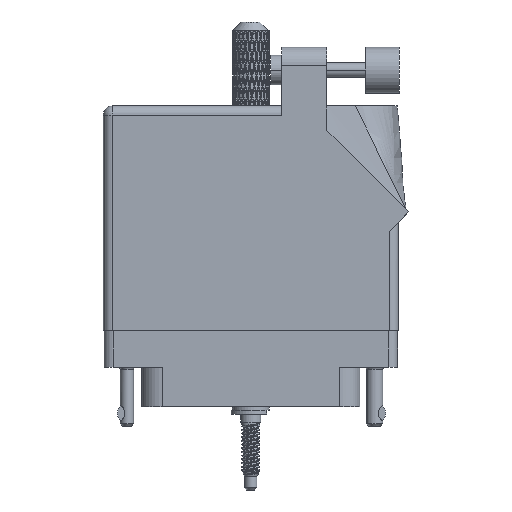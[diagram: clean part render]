
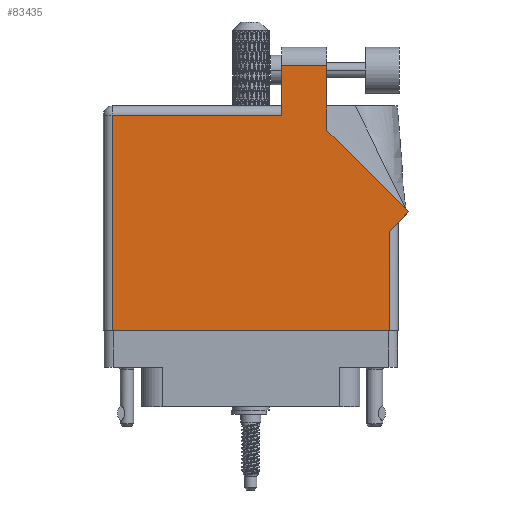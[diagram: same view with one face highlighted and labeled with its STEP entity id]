
A CAD part, front view. The second image highlights one B-rep face of the part: STEP entity #83435.
In plain terms, the highlighted face is planar.
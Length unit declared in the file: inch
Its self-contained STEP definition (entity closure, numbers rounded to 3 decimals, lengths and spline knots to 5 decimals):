
#87 = DIRECTION ( 'NONE',  ( 0., 0., -1. ) ) ;
#1238 = CARTESIAN_POINT ( 'NONE',  ( -0.943, 1.368, 0.455 ) ) ;
#1897 = VERTEX_POINT ( 'NONE', #28675 ) ;
#4050 = VERTEX_POINT ( 'NONE', #73638 ) ;
#4842 = EDGE_CURVE ( 'NONE', #1897, #29199, #67476, .T. ) ;
#5436 = DIRECTION ( 'NONE',  ( 0., 1., 0. ) ) ;
#7036 = ORIENTED_EDGE ( 'NONE', *, *, #47555, .T. ) ;
#7184 = LINE ( 'NONE', #101073, #16944 ) ;
#7627 = LINE ( 'NONE', #17118, #114527 ) ;
#7717 = DIRECTION ( 'NONE',  ( 0.707, 0.707, 0. ) ) ;
#9039 = VECTOR ( 'NONE', #5436, 39.37008 ) ;
#9808 = CARTESIAN_POINT ( 'NONE',  ( -1.005, 1.43, 0.455 ) ) ;
#15026 = VECTOR ( 'NONE', #84404, 39.37008 ) ;
#16944 = VECTOR ( 'NONE', #48210, 39.37008 ) ;
#17118 = CARTESIAN_POINT ( 'NONE',  ( 0.212, 1.43, 0.455 ) ) ;
#23629 = DIRECTION ( 'NONE',  ( 0., 1., 0. ) ) ;
#24159 = VERTEX_POINT ( 'NONE', #89718 ) ;
#24537 = EDGE_LOOP ( 'NONE', ( #7036, #66713, #81963, #40943, #89921, #25358, #95465, #99222, #57016 ) ) ;
#25358 = ORIENTED_EDGE ( 'NONE', *, *, #101197, .T. ) ;
#25859 = EDGE_CURVE ( 'NONE', #4050, #98365, #52923, .T. ) ;
#28675 = CARTESIAN_POINT ( 'NONE',  ( 0.212, 1.368, 0.455 ) ) ;
#29199 = VERTEX_POINT ( 'NONE', #1238 ) ;
#29390 = VERTEX_POINT ( 'NONE', #30710 ) ;
#29556 = EDGE_CURVE ( 'NONE', #29390, #1897, #7627, .T. ) ;
#30710 = CARTESIAN_POINT ( 'NONE',  ( 0.212, 1.705, 0.455 ) ) ;
#32322 = EDGE_CURVE ( 'NONE', #98365, #46793, #7184, .T. ) ;
#33347 = EDGE_CURVE ( 'NONE', #80316, #29390, #57015, .T. ) ;
#38463 = DIRECTION ( 'NONE',  ( -1., 0., 0. ) ) ;
#39358 = CARTESIAN_POINT ( 'NONE',  ( -0.943, -0.1, 0.455 ) ) ;
#40943 = ORIENTED_EDGE ( 'NONE', *, *, #4842, .T. ) ;
#42503 = LINE ( 'NONE', #50650, #74546 ) ;
#45902 = CARTESIAN_POINT ( 'NONE',  ( -1.005, -0.1, 0.455 ) ) ;
#46274 = DIRECTION ( 'NONE',  ( -1., 0., 0. ) ) ;
#46793 = VERTEX_POINT ( 'NONE', #74766 ) ;
#47456 = CARTESIAN_POINT ( 'NONE',  ( 0.212, 1.705, 0.455 ) ) ;
#47555 = EDGE_CURVE ( 'NONE', #46793, #80316, #57647, .T. ) ;
#48166 = CARTESIAN_POINT ( 'NONE',  ( 0.943, -0.1, 0.455 ) ) ;
#48210 = DIRECTION ( 'NONE',  ( -0.707, 0.707, 0. ) ) ;
#50650 = CARTESIAN_POINT ( 'NONE',  ( 0.943, 0.637, 0.455 ) ) ;
#52337 = CARTESIAN_POINT ( 'NONE',  ( 1.005, 0.637, 0.455 ) ) ;
#52837 = VECTOR ( 'NONE', #46274, 39.37008 ) ;
#52916 = LINE ( 'NONE', #45902, #77873 ) ;
#52923 = LINE ( 'NONE', #52337, #58541 ) ;
#53449 = EDGE_CURVE ( 'NONE', #29199, #24159, #88549, .T. ) ;
#53656 = VERTEX_POINT ( 'NONE', #48166 ) ;
#57015 = LINE ( 'NONE', #47456, #52837 ) ;
#57016 = ORIENTED_EDGE ( 'NONE', *, *, #32322, .T. ) ;
#57095 = CARTESIAN_POINT ( 'NONE',  ( 0.519, 1.26442, 0.455 ) ) ;
#57647 = LINE ( 'NONE', #57095, #9039 ) ;
#58541 = VECTOR ( 'NONE', #7717, 39.37008 ) ;
#61053 = CARTESIAN_POINT ( 'NONE',  ( 1.07571, 0.70771, 0.455 ) ) ;
#62543 = PLANE ( 'NONE',  #106112 ) ;
#66713 = ORIENTED_EDGE ( 'NONE', *, *, #33347, .T. ) ;
#67476 = LINE ( 'NONE', #81575, #82774 ) ;
#73638 = CARTESIAN_POINT ( 'NONE',  ( 0.943, 0.575, 0.455 ) ) ;
#74546 = VECTOR ( 'NONE', #23629, 39.37008 ) ;
#74766 = CARTESIAN_POINT ( 'NONE',  ( 0.519, 1.26442, 0.455 ) ) ;
#75378 = FACE_OUTER_BOUND ( 'NONE', #24537, .T. ) ;
#77873 = VECTOR ( 'NONE', #92595, 39.37008 ) ;
#80316 = VERTEX_POINT ( 'NONE', #106563 ) ;
#81575 = CARTESIAN_POINT ( 'NONE',  ( -1.005, 1.368, 0.455 ) ) ;
#81963 = ORIENTED_EDGE ( 'NONE', *, *, #29556, .T. ) ;
#82774 = VECTOR ( 'NONE', #38463, 39.37008 ) ;
#83435 = ADVANCED_FACE ( 'NONE', ( #75378 ), #62543, .F. ) ;
#84404 = DIRECTION ( 'NONE',  ( 0., -1., 0. ) ) ;
#88549 = LINE ( 'NONE', #39358, #15026 ) ;
#89718 = CARTESIAN_POINT ( 'NONE',  ( -0.943, -0.1, 0.455 ) ) ;
#89921 = ORIENTED_EDGE ( 'NONE', *, *, #53449, .T. ) ;
#92595 = DIRECTION ( 'NONE',  ( 1., 0., 0. ) ) ;
#95465 = ORIENTED_EDGE ( 'NONE', *, *, #95987, .T. ) ;
#95840 = DIRECTION ( 'NONE',  ( 0., -1., 0. ) ) ;
#95987 = EDGE_CURVE ( 'NONE', #53656, #4050, #42503, .T. ) ;
#98365 = VERTEX_POINT ( 'NONE', #61053 ) ;
#99222 = ORIENTED_EDGE ( 'NONE', *, *, #25859, .T. ) ;
#101073 = CARTESIAN_POINT ( 'NONE',  ( 1.07571, 0.70771, 0.455 ) ) ;
#101197 = EDGE_CURVE ( 'NONE', #24159, #53656, #52916, .T. ) ;
#106112 = AXIS2_PLACEMENT_3D ( 'NONE', #9808, #87, #106808 ) ;
#106563 = CARTESIAN_POINT ( 'NONE',  ( 0.519, 1.705, 0.455 ) ) ;
#106808 = DIRECTION ( 'NONE',  ( -1., 0., 0. ) ) ;
#114527 = VECTOR ( 'NONE', #95840, 39.37008 ) ;
